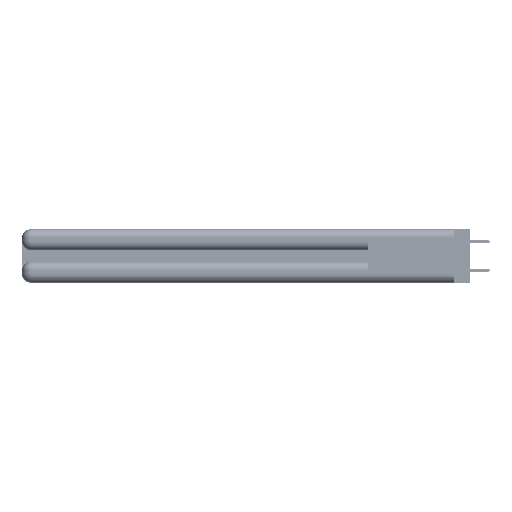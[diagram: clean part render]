
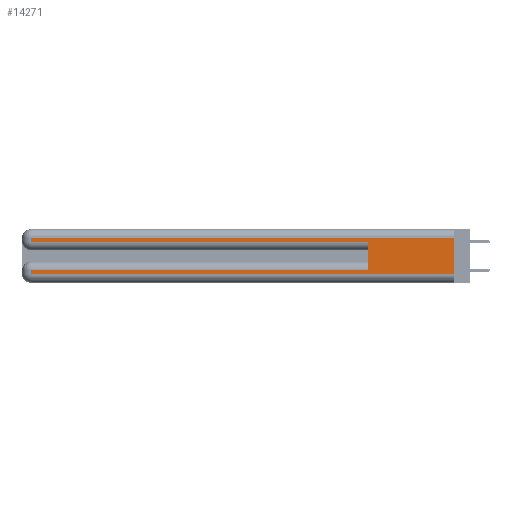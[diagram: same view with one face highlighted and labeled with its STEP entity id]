
A CAD part, left-side view. The second image highlights one B-rep face of the part: STEP entity #14271.
In plain terms, the highlighted planar face has unit normal (-1, 0, 0).
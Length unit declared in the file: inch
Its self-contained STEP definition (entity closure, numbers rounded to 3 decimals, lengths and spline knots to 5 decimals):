
#1091 = VERTEX_POINT ( 'NONE', #45623 ) ;
#1372 = CARTESIAN_POINT ( 'NONE',  ( 0., 2.94, 0.06 ) ) ;
#1999 = ORIENTED_EDGE ( 'NONE', *, *, #46370, .T. ) ;
#4681 = DIRECTION ( 'NONE',  ( 1., 0., 0. ) ) ;
#4756 = VECTOR ( 'NONE', #45239, 39.37008 ) ;
#5214 = EDGE_CURVE ( 'NONE', #41726, #56199, #35733, .T. ) ;
#5490 = CARTESIAN_POINT ( 'NONE',  ( 0., 0., 0.085 ) ) ;
#7953 = CARTESIAN_POINT ( 'NONE',  ( 0., 0., 0.31 ) ) ;
#8271 = ORIENTED_EDGE ( 'NONE', *, *, #5214, .F. ) ;
#9632 = DIRECTION ( 'NONE',  ( 0., 0., -1. ) ) ;
#10556 = LINE ( 'NONE', #12784, #40644 ) ;
#11593 = CARTESIAN_POINT ( 'NONE',  ( 0., 2.94, 0.085 ) ) ;
#11967 = ORIENTED_EDGE ( 'NONE', *, *, #34382, .T. ) ;
#12784 = CARTESIAN_POINT ( 'NONE',  ( 0., 2.94, 0.37 ) ) ;
#12785 = DIRECTION ( 'NONE',  ( 0., 0., -1. ) ) ;
#12945 = CARTESIAN_POINT ( 'NONE',  ( 0., 0.6, 0.085 ) ) ;
#13570 = LINE ( 'NONE', #14309, #14220 ) ;
#13685 = DIRECTION ( 'NONE',  ( 0., 1., 0. ) ) ;
#14220 = VECTOR ( 'NONE', #14502, 39.37008 ) ;
#14271 = ADVANCED_FACE ( 'NONE', ( #51797 ), #26746, .F. ) ;
#14309 = CARTESIAN_POINT ( 'NONE',  ( 0., 0., 0.31 ) ) ;
#14502 = DIRECTION ( 'NONE',  ( 0., 1., 0. ) ) ;
#14510 = AXIS2_PLACEMENT_3D ( 'NONE', #56280, #4681, #34776 ) ;
#14543 = LINE ( 'NONE', #36497, #54118 ) ;
#16334 = VECTOR ( 'NONE', #12785, 39.37008 ) ;
#17180 = EDGE_CURVE ( 'NONE', #35808, #29631, #10556, .T. ) ;
#18858 = DIRECTION ( 'NONE',  ( 0., 0., 1. ) ) ;
#20300 = EDGE_CURVE ( 'NONE', #38289, #25186, #43743, .T. ) ;
#21381 = DIRECTION ( 'NONE',  ( 0., 0., -1. ) ) ;
#21552 = EDGE_CURVE ( 'NONE', #41726, #35808, #36040, .T. ) ;
#22712 = CARTESIAN_POINT ( 'NONE',  ( 0., 0., 0.285 ) ) ;
#23759 = ORIENTED_EDGE ( 'NONE', *, *, #25788, .T. ) ;
#25186 = VERTEX_POINT ( 'NONE', #26259 ) ;
#25764 = CARTESIAN_POINT ( 'NONE',  ( 0., 2.94, 0.37 ) ) ;
#25788 = EDGE_CURVE ( 'NONE', #50766, #1091, #29288, .T. ) ;
#25983 = ORIENTED_EDGE ( 'NONE', *, *, #21552, .T. ) ;
#26259 = CARTESIAN_POINT ( 'NONE',  ( 0., 0., 0.06 ) ) ;
#26547 = LINE ( 'NONE', #22712, #4756 ) ;
#26746 = PLANE ( 'NONE',  #14510 ) ;
#28521 = VECTOR ( 'NONE', #13685, 39.37008 ) ;
#29288 = LINE ( 'NONE', #25764, #16334 ) ;
#29631 = VERTEX_POINT ( 'NONE', #1372 ) ;
#30065 = VECTOR ( 'NONE', #9632, 39.37008 ) ;
#32016 = ORIENTED_EDGE ( 'NONE', *, *, #40336, .T. ) ;
#34382 = EDGE_CURVE ( 'NONE', #1091, #56199, #26547, .T. ) ;
#34776 = DIRECTION ( 'NONE',  ( 0., 0., -1. ) ) ;
#35733 = LINE ( 'NONE', #53398, #38498 ) ;
#35808 = VERTEX_POINT ( 'NONE', #11593 ) ;
#36040 = LINE ( 'NONE', #5490, #28521 ) ;
#36497 = CARTESIAN_POINT ( 'NONE',  ( 0., 0., 0.06 ) ) ;
#38289 = VERTEX_POINT ( 'NONE', #7953 ) ;
#38498 = VECTOR ( 'NONE', #18858, 39.37008 ) ;
#40336 = EDGE_CURVE ( 'NONE', #29631, #25186, #14543, .T. ) ;
#40644 = VECTOR ( 'NONE', #21381, 39.37008 ) ;
#41609 = ORIENTED_EDGE ( 'NONE', *, *, #20300, .F. ) ;
#41726 = VERTEX_POINT ( 'NONE', #12945 ) ;
#42955 = ORIENTED_EDGE ( 'NONE', *, *, #17180, .T. ) ;
#43743 = LINE ( 'NONE', #53128, #30065 ) ;
#45239 = DIRECTION ( 'NONE',  ( 0., -1., 0. ) ) ;
#45297 = DIRECTION ( 'NONE',  ( 0., -1., 0. ) ) ;
#45623 = CARTESIAN_POINT ( 'NONE',  ( 0., 2.94, 0.285 ) ) ;
#46370 = EDGE_CURVE ( 'NONE', #38289, #50766, #13570, .T. ) ;
#50254 = CARTESIAN_POINT ( 'NONE',  ( 0., 2.94, 0.31 ) ) ;
#50766 = VERTEX_POINT ( 'NONE', #50254 ) ;
#51636 = EDGE_LOOP ( 'NONE', ( #41609, #1999, #23759, #11967, #8271, #25983, #42955, #32016 ) ) ;
#51797 = FACE_OUTER_BOUND ( 'NONE', #51636, .T. ) ;
#53128 = CARTESIAN_POINT ( 'NONE',  ( 0., 0., 0.37 ) ) ;
#53398 = CARTESIAN_POINT ( 'NONE',  ( 0., 0.6, 0.145 ) ) ;
#54118 = VECTOR ( 'NONE', #45297, 39.37008 ) ;
#55231 = CARTESIAN_POINT ( 'NONE',  ( 0., 0.6, 0.285 ) ) ;
#56199 = VERTEX_POINT ( 'NONE', #55231 ) ;
#56280 = CARTESIAN_POINT ( 'NONE',  ( 0., 0., 0.37 ) ) ;
